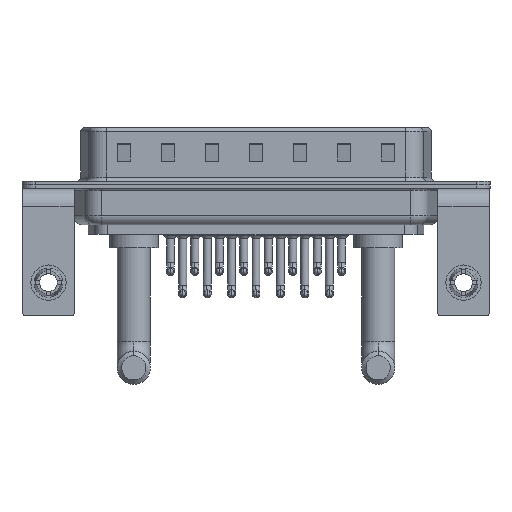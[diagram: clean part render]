
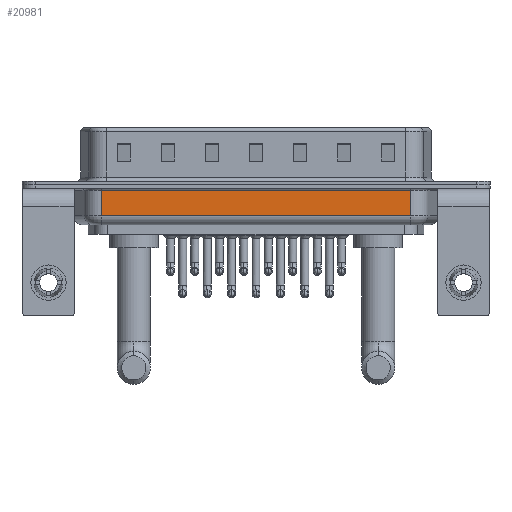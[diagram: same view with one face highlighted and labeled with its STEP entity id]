
A CAD part, front view. The second image highlights one B-rep face of the part: STEP entity #20981.
In plain terms, the highlighted planar face has unit normal (0, -1, 0).
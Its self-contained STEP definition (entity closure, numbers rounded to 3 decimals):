
#286 = PLANE ( 'NONE',  #25005 ) ;
#1132 = ORIENTED_EDGE ( 'NONE', *, *, #15080, .F. ) ;
#2155 = ORIENTED_EDGE ( 'NONE', *, *, #8385, .T. ) ;
#2210 = CARTESIAN_POINT ( 'NONE',  ( 6.006, -5.35, -3.5 ) ) ;
#2470 = CARTESIAN_POINT ( 'NONE',  ( 6.006, -5.35, -4.5 ) ) ;
#2601 = DIRECTION ( 'NONE',  ( 0., 1., 0. ) ) ;
#3060 = CARTESIAN_POINT ( 'NONE',  ( 41.044, -5.35, -0.65 ) ) ;
#3061 = VECTOR ( 'NONE', #22672, 1000. ) ;
#3678 = VERTEX_POINT ( 'NONE', #3060 ) ;
#4433 = LINE ( 'NONE', #27101, #5719 ) ;
#5719 = VECTOR ( 'NONE', #6238, 1000. ) ;
#5824 = DIRECTION ( 'NONE',  ( 0., 0., 1. ) ) ;
#6238 = DIRECTION ( 'NONE',  ( 0., 0., 1. ) ) ;
#6898 = CARTESIAN_POINT ( 'NONE',  ( 6.006, -5.35, -3.5 ) ) ;
#8247 = CARTESIAN_POINT ( 'NONE',  ( 6.006, -5.35, -0.65 ) ) ;
#8385 = EDGE_CURVE ( 'NONE', #12907, #3678, #14485, .T. ) ;
#8427 = CARTESIAN_POINT ( 'NONE',  ( 41.044, -5.35, -3.5 ) ) ;
#9300 = VECTOR ( 'NONE', #23798, 1000. ) ;
#12335 = CARTESIAN_POINT ( 'NONE',  ( 6.006, -5.35, -0.65 ) ) ;
#12902 = DIRECTION ( 'NONE',  ( 0., 0., 1. ) ) ;
#12907 = VERTEX_POINT ( 'NONE', #8427 ) ;
#14349 = CARTESIAN_POINT ( 'NONE',  ( 41.044, -5.35, -4.5 ) ) ;
#14485 = LINE ( 'NONE', #14349, #22589 ) ;
#15080 = EDGE_CURVE ( 'NONE', #20965, #19961, #4433, .T. ) ;
#16088 = ORIENTED_EDGE ( 'NONE', *, *, #23237, .T. ) ;
#16133 = ORIENTED_EDGE ( 'NONE', *, *, #20782, .T. ) ;
#16895 = FACE_OUTER_BOUND ( 'NONE', #18141, .T. ) ;
#18141 = EDGE_LOOP ( 'NONE', ( #1132, #16088, #2155, #16133 ) ) ;
#19272 = LINE ( 'NONE', #6898, #9300 ) ;
#19961 = VERTEX_POINT ( 'NONE', #12335 ) ;
#20782 = EDGE_CURVE ( 'NONE', #3678, #19961, #26642, .T. ) ;
#20965 = VERTEX_POINT ( 'NONE', #2210 ) ;
#20981 = ADVANCED_FACE ( 'NONE', ( #16895 ), #286, .F. ) ;
#22589 = VECTOR ( 'NONE', #5824, 1000. ) ;
#22672 = DIRECTION ( 'NONE',  ( -1., 0., 0. ) ) ;
#23237 = EDGE_CURVE ( 'NONE', #20965, #12907, #19272, .T. ) ;
#23798 = DIRECTION ( 'NONE',  ( 1., 0., 0. ) ) ;
#25005 = AXIS2_PLACEMENT_3D ( 'NONE', #2470, #2601, #12902 ) ;
#26642 = LINE ( 'NONE', #8247, #3061 ) ;
#27101 = CARTESIAN_POINT ( 'NONE',  ( 6.006, -5.35, -4.5 ) ) ;
